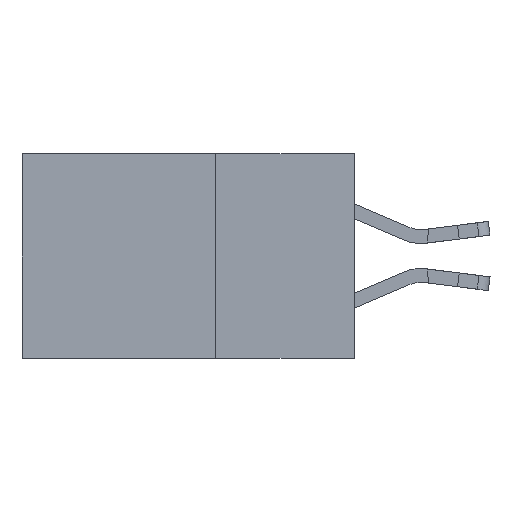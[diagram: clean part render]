
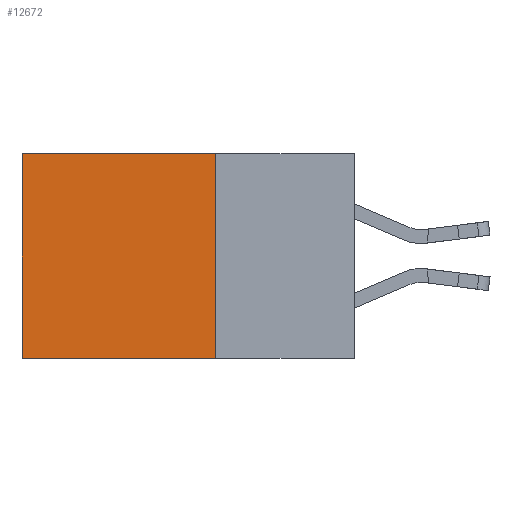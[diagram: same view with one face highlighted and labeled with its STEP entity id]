
A CAD part, left-side view. The second image highlights one B-rep face of the part: STEP entity #12672.
In plain terms, the highlighted planar face has unit normal (-1, 0, 0).
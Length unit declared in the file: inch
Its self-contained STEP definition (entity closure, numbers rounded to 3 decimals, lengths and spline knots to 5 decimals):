
#26 = VERTEX_POINT ( 'NONE', #11542 ) ;
#779 = LINE ( 'NONE', #18446, #14448 ) ;
#1572 = CARTESIAN_POINT ( 'NONE',  ( 0.2615, 0.25, -0.37 ) ) ;
#1590 = VECTOR ( 'NONE', #10004, 39.37008 ) ;
#2418 = VECTOR ( 'NONE', #17439, 39.37008 ) ;
#3517 = DIRECTION ( 'NONE',  ( 0., 0., -1. ) ) ;
#3546 = VERTEX_POINT ( 'NONE', #8643 ) ;
#3982 = EDGE_CURVE ( 'NONE', #26, #17052, #779, .T. ) ;
#5412 = CARTESIAN_POINT ( 'NONE',  ( 0.2615, 0.25, -0.37 ) ) ;
#7190 = AXIS2_PLACEMENT_3D ( 'NONE', #5412, #7218, #19482 ) ;
#7218 = DIRECTION ( 'NONE',  ( 1., 0., 0. ) ) ;
#8233 = EDGE_CURVE ( 'NONE', #17433, #3546, #11084, .T. ) ;
#8643 = CARTESIAN_POINT ( 'NONE',  ( 0.2615, 0.6, -0.37 ) ) ;
#10004 = DIRECTION ( 'NONE',  ( 0., 1., 0. ) ) ;
#10203 = ORIENTED_EDGE ( 'NONE', *, *, #15704, .T. ) ;
#11084 = LINE ( 'NONE', #17073, #1590 ) ;
#11542 = CARTESIAN_POINT ( 'NONE',  ( 0.2615, 0.25, 0. ) ) ;
#12672 = ADVANCED_FACE ( 'NONE', ( #16491 ), #14211, .F. ) ;
#12988 = CARTESIAN_POINT ( 'NONE',  ( 0.2615, 0.6, 0. ) ) ;
#14211 = PLANE ( 'NONE',  #7190 ) ;
#14448 = VECTOR ( 'NONE', #15025, 39.37008 ) ;
#15025 = DIRECTION ( 'NONE',  ( 0., 1., 0. ) ) ;
#15291 = LINE ( 'NONE', #15887, #19932 ) ;
#15326 = ORIENTED_EDGE ( 'NONE', *, *, #3982, .T. ) ;
#15704 = EDGE_CURVE ( 'NONE', #17052, #3546, #15291, .T. ) ;
#15887 = CARTESIAN_POINT ( 'NONE',  ( 0.2615, 0.6, -0.37 ) ) ;
#16491 = FACE_OUTER_BOUND ( 'NONE', #22728, .T. ) ;
#17052 = VERTEX_POINT ( 'NONE', #12988 ) ;
#17073 = CARTESIAN_POINT ( 'NONE',  ( 0.2615, 0.25, -0.37 ) ) ;
#17400 = ORIENTED_EDGE ( 'NONE', *, *, #18132, .F. ) ;
#17433 = VERTEX_POINT ( 'NONE', #20990 ) ;
#17439 = DIRECTION ( 'NONE',  ( 0., 0., -1. ) ) ;
#18132 = EDGE_CURVE ( 'NONE', #26, #17433, #20098, .T. ) ;
#18446 = CARTESIAN_POINT ( 'NONE',  ( 0.2615, 0.25, 0. ) ) ;
#19482 = DIRECTION ( 'NONE',  ( 0., 0., -1. ) ) ;
#19932 = VECTOR ( 'NONE', #3517, 39.37008 ) ;
#20098 = LINE ( 'NONE', #1572, #2418 ) ;
#20665 = ORIENTED_EDGE ( 'NONE', *, *, #8233, .F. ) ;
#20990 = CARTESIAN_POINT ( 'NONE',  ( 0.2615, 0.25, -0.37 ) ) ;
#22728 = EDGE_LOOP ( 'NONE', ( #10203, #20665, #17400, #15326 ) ) ;
